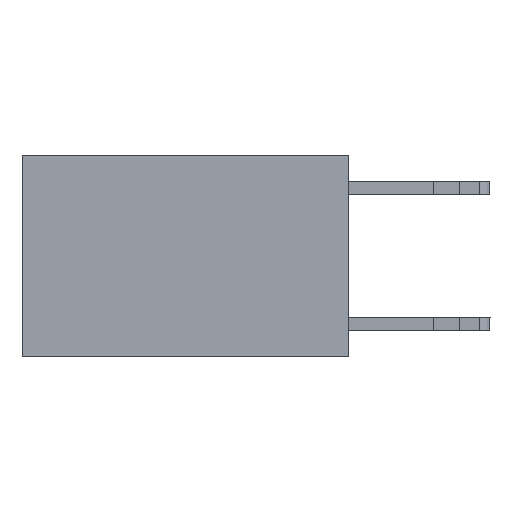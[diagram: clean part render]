
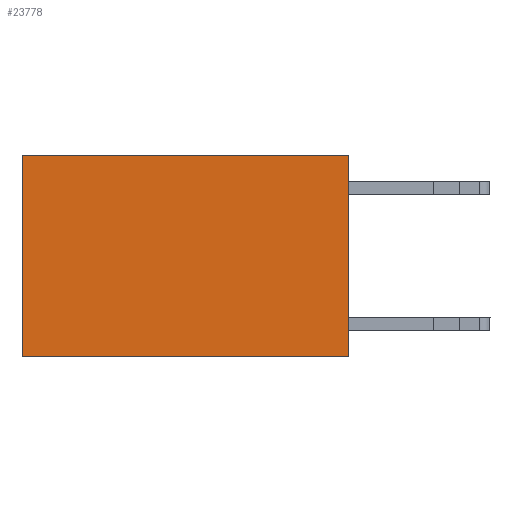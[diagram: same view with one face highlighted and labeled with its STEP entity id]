
A CAD part, left-side view. The second image highlights one B-rep face of the part: STEP entity #23778.
In plain terms, the highlighted planar face has unit normal (-1, 0, 0).
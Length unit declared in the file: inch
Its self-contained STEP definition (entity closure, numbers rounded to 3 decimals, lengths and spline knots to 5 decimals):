
#175 = VERTEX_POINT ( 'NONE', #1520 ) ;
#1132 = LINE ( 'NONE', #8833, #23439 ) ;
#1520 = CARTESIAN_POINT ( 'NONE',  ( 0.2625, 0.6, 0. ) ) ;
#3410 = LINE ( 'NONE', #22609, #13290 ) ;
#3425 = CARTESIAN_POINT ( 'NONE',  ( 0.2625, 0., 0. ) ) ;
#3949 = VERTEX_POINT ( 'NONE', #3425 ) ;
#5669 = FACE_OUTER_BOUND ( 'NONE', #9615, .T. ) ;
#6941 = CARTESIAN_POINT ( 'NONE',  ( 0.2625, 0., -0.37 ) ) ;
#8540 = VERTEX_POINT ( 'NONE', #12508 ) ;
#8833 = CARTESIAN_POINT ( 'NONE',  ( 0.2625, 0.6, 0. ) ) ;
#9127 = EDGE_CURVE ( 'NONE', #175, #8540, #1132, .T. ) ;
#9355 = ORIENTED_EDGE ( 'NONE', *, *, #9127, .T. ) ;
#9615 = EDGE_LOOP ( 'NONE', ( #9355, #20032, #21472, #12946 ) ) ;
#10950 = VECTOR ( 'NONE', #23726, 39.37008 ) ;
#12456 = DIRECTION ( 'NONE',  ( 0., 0., -1. ) ) ;
#12508 = CARTESIAN_POINT ( 'NONE',  ( 0.2625, 0.6, -0.37 ) ) ;
#12946 = ORIENTED_EDGE ( 'NONE', *, *, #26484, .T. ) ;
#13290 = VECTOR ( 'NONE', #18467, 39.37008 ) ;
#13626 = VECTOR ( 'NONE', #25730, 39.37008 ) ;
#17150 = LINE ( 'NONE', #6941, #10950 ) ;
#18467 = DIRECTION ( 'NONE',  ( 0., 0., -1. ) ) ;
#18485 = LINE ( 'NONE', #23804, #13626 ) ;
#20032 = ORIENTED_EDGE ( 'NONE', *, *, #23344, .F. ) ;
#20583 = CARTESIAN_POINT ( 'NONE',  ( 0.2625, 0., -0.37 ) ) ;
#20754 = CARTESIAN_POINT ( 'NONE',  ( 0.2625, 0., 0. ) ) ;
#21402 = AXIS2_PLACEMENT_3D ( 'NONE', #20754, #24974, #12456 ) ;
#21472 = ORIENTED_EDGE ( 'NONE', *, *, #23705, .F. ) ;
#22609 = CARTESIAN_POINT ( 'NONE',  ( 0.2625, 0., 0. ) ) ;
#23344 = EDGE_CURVE ( 'NONE', #24205, #8540, #17150, .T. ) ;
#23439 = VECTOR ( 'NONE', #23482, 39.37008 ) ;
#23482 = DIRECTION ( 'NONE',  ( 0., 0., -1. ) ) ;
#23705 = EDGE_CURVE ( 'NONE', #3949, #24205, #3410, .T. ) ;
#23726 = DIRECTION ( 'NONE',  ( 0., 1., 0. ) ) ;
#23778 = ADVANCED_FACE ( 'NONE', ( #5669 ), #24877, .F. ) ;
#23804 = CARTESIAN_POINT ( 'NONE',  ( 0.2625, 0., 0. ) ) ;
#24205 = VERTEX_POINT ( 'NONE', #20583 ) ;
#24877 = PLANE ( 'NONE',  #21402 ) ;
#24974 = DIRECTION ( 'NONE',  ( 1., 0., 0. ) ) ;
#25730 = DIRECTION ( 'NONE',  ( 0., 1., 0. ) ) ;
#26484 = EDGE_CURVE ( 'NONE', #3949, #175, #18485, .T. ) ;
